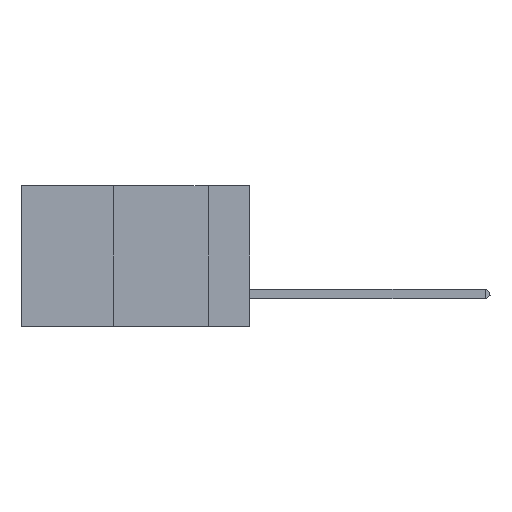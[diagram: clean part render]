
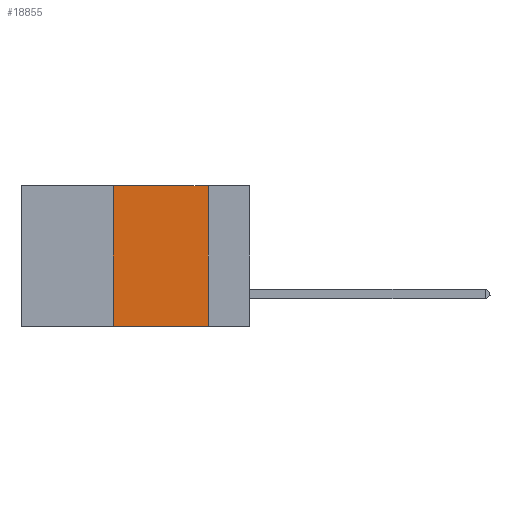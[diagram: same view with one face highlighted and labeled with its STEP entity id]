
A CAD part, left-side view. The second image highlights one B-rep face of the part: STEP entity #18855.
In plain terms, the highlighted planar face has unit normal (-1, 0, 0).
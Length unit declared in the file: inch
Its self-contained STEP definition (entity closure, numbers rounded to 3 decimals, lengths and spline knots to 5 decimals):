
#1756 = ORIENTED_EDGE ( 'NONE', *, *, #3105, .F. ) ;
#1806 = VERTEX_POINT ( 'NONE', #5557 ) ;
#1832 = ORIENTED_EDGE ( 'NONE', *, *, #7343, .F. ) ;
#1938 = DIRECTION ( 'NONE',  ( 0., -1., 0. ) ) ;
#2250 = CARTESIAN_POINT ( 'NONE',  ( 0., 0.6, 0. ) ) ;
#2257 = VERTEX_POINT ( 'NONE', #5957 ) ;
#3105 = EDGE_CURVE ( 'NONE', #13514, #15286, #12747, .T. ) ;
#3224 = CARTESIAN_POINT ( 'NONE',  ( 0., 0.6, -0.37 ) ) ;
#3897 = PLANE ( 'NONE',  #15824 ) ;
#4287 = DIRECTION ( 'NONE',  ( 1., 0., 0. ) ) ;
#5557 = CARTESIAN_POINT ( 'NONE',  ( 0., 0.11, 0. ) ) ;
#5654 = ORIENTED_EDGE ( 'NONE', *, *, #16274, .T. ) ;
#5957 = CARTESIAN_POINT ( 'NONE',  ( 0., 0.11, -0.37 ) ) ;
#5969 = EDGE_CURVE ( 'NONE', #15286, #1806, #16321, .T. ) ;
#6806 = CARTESIAN_POINT ( 'NONE',  ( 0., 0.36, 0. ) ) ;
#7018 = DIRECTION ( 'NONE',  ( 0., 0., -1. ) ) ;
#7343 = EDGE_CURVE ( 'NONE', #1806, #2257, #14455, .T. ) ;
#7457 = VECTOR ( 'NONE', #1938, 39.37008 ) ;
#8762 = VECTOR ( 'NONE', #15759, 39.37008 ) ;
#10486 = VECTOR ( 'NONE', #13684, 39.37008 ) ;
#11201 = CARTESIAN_POINT ( 'NONE',  ( 0., 0.36, 0. ) ) ;
#12054 = ORIENTED_EDGE ( 'NONE', *, *, #5969, .F. ) ;
#12747 = LINE ( 'NONE', #6806, #8762 ) ;
#13177 = EDGE_LOOP ( 'NONE', ( #1832, #12054, #1756, #5654 ) ) ;
#13514 = VERTEX_POINT ( 'NONE', #14189 ) ;
#13684 = DIRECTION ( 'NONE',  ( 0., -1., 0. ) ) ;
#13846 = CARTESIAN_POINT ( 'NONE',  ( 0., 0.6, 0. ) ) ;
#14189 = CARTESIAN_POINT ( 'NONE',  ( 0., 0.36, -0.37 ) ) ;
#14455 = LINE ( 'NONE', #19012, #17953 ) ;
#15286 = VERTEX_POINT ( 'NONE', #11201 ) ;
#15759 = DIRECTION ( 'NONE',  ( 0., 0., 1. ) ) ;
#15762 = FACE_OUTER_BOUND ( 'NONE', #13177, .T. ) ;
#15824 = AXIS2_PLACEMENT_3D ( 'NONE', #2250, #4287, #17624 ) ;
#16274 = EDGE_CURVE ( 'NONE', #13514, #2257, #18416, .T. ) ;
#16321 = LINE ( 'NONE', #13846, #7457 ) ;
#17624 = DIRECTION ( 'NONE',  ( 0., 0., -1. ) ) ;
#17953 = VECTOR ( 'NONE', #7018, 39.37008 ) ;
#18416 = LINE ( 'NONE', #3224, #10486 ) ;
#18855 = ADVANCED_FACE ( 'NONE', ( #15762 ), #3897, .F. ) ;
#19012 = CARTESIAN_POINT ( 'NONE',  ( 0., 0.11, 0. ) ) ;
